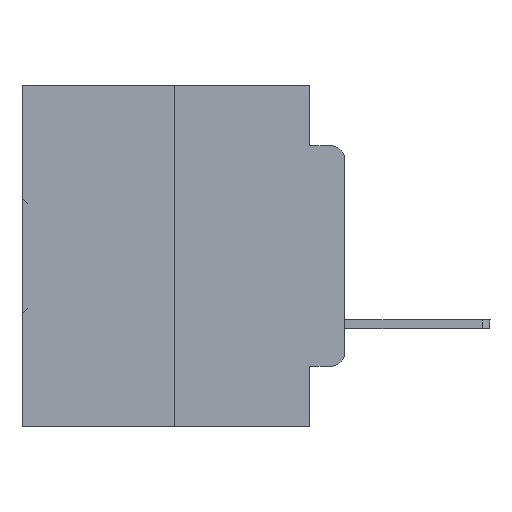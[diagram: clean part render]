
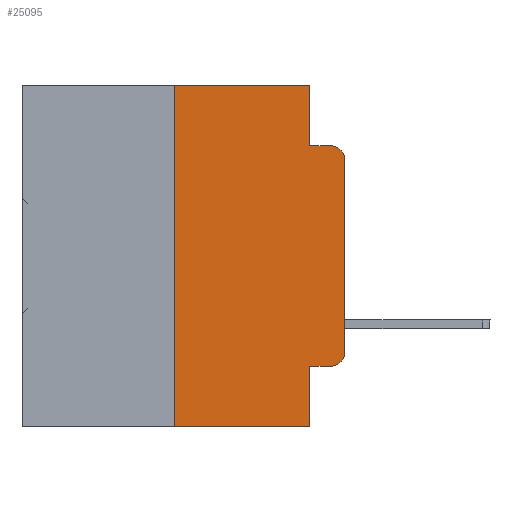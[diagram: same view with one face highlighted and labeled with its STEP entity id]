
A CAD part, left-side view. The second image highlights one B-rep face of the part: STEP entity #25095.
In plain terms, the highlighted planar face has unit normal (-1, 0, 0).
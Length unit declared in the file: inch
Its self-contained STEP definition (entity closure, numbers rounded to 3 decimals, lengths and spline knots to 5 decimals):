
#17 = VERTEX_POINT ( 'NONE', #32914 ) ;
#161 = DIRECTION ( 'NONE',  ( 0., 0., 1. ) ) ;
#197 = LINE ( 'NONE', #3133, #27004 ) ;
#233 = VERTEX_POINT ( 'NONE', #13519 ) ;
#1277 = AXIS2_PLACEMENT_3D ( 'NONE', #22930, #14975, #9777 ) ;
#1588 = CIRCLE ( 'NONE', #32548, 0.02 ) ;
#2910 = CARTESIAN_POINT ( 'NONE',  ( 0., 0.02, -0.1085 ) ) ;
#2919 = VERTEX_POINT ( 'NONE', #33240 ) ;
#2960 = CARTESIAN_POINT ( 'NONE',  ( 0., 0.25, 0. ) ) ;
#3133 = CARTESIAN_POINT ( 'NONE',  ( 0., 0., 0. ) ) ;
#3198 = VECTOR ( 'NONE', #15450, 39.37008 ) ;
#3259 = VERTEX_POINT ( 'NONE', #22315 ) ;
#3593 = EDGE_CURVE ( 'NONE', #28113, #3259, #18991, .T. ) ;
#3687 = CARTESIAN_POINT ( 'NONE',  ( 0., 0.473, 0. ) ) ;
#3763 = CARTESIAN_POINT ( 'NONE',  ( 0., 0.051, 0. ) ) ;
#4134 = CARTESIAN_POINT ( 'NONE',  ( 0., 0.051, -0.4115 ) ) ;
#4249 = AXIS2_PLACEMENT_3D ( 'NONE', #3687, #21856, #28205 ) ;
#4775 = DIRECTION ( 'NONE',  ( 0., -1., 0. ) ) ;
#5702 = CIRCLE ( 'NONE', #1277, 0.02 ) ;
#6539 = ORIENTED_EDGE ( 'NONE', *, *, #26640, .T. ) ;
#8245 = VERTEX_POINT ( 'NONE', #19595 ) ;
#8255 = EDGE_LOOP ( 'NONE', ( #6539, #17867, #20462, #9425, #28449, #27258, #11846, #21145, #8725, #27569 ) ) ;
#8432 = VERTEX_POINT ( 'NONE', #2960 ) ;
#8687 = CARTESIAN_POINT ( 'NONE',  ( 0., 0.02, -0.4115 ) ) ;
#8717 = FACE_OUTER_BOUND ( 'NONE', #8255, .T. ) ;
#8725 = ORIENTED_EDGE ( 'NONE', *, *, #16776, .T. ) ;
#9425 = ORIENTED_EDGE ( 'NONE', *, *, #13124, .F. ) ;
#9511 = EDGE_CURVE ( 'NONE', #33677, #17, #5702, .T. ) ;
#9608 = LINE ( 'NONE', #30897, #21952 ) ;
#9777 = DIRECTION ( 'NONE',  ( 0., 0., -1. ) ) ;
#9856 = LINE ( 'NONE', #20417, #18588 ) ;
#10170 = EDGE_CURVE ( 'NONE', #8245, #8432, #16103, .T. ) ;
#10611 = DIRECTION ( 'NONE',  ( 0., 0., -1. ) ) ;
#10688 = DIRECTION ( 'NONE',  ( 0., 0., -1. ) ) ;
#10712 = DIRECTION ( 'NONE',  ( 0., -1., 0. ) ) ;
#10887 = CARTESIAN_POINT ( 'NONE',  ( 0., 0.25, 0. ) ) ;
#11199 = DIRECTION ( 'NONE',  ( 0., 0., -1. ) ) ;
#11297 = PLANE ( 'NONE',  #4249 ) ;
#11846 = ORIENTED_EDGE ( 'NONE', *, *, #22435, .T. ) ;
#12479 = LINE ( 'NONE', #22522, #3198 ) ;
#13124 = EDGE_CURVE ( 'NONE', #233, #30140, #33976, .T. ) ;
#13519 = CARTESIAN_POINT ( 'NONE',  ( 0., 0.051, 0. ) ) ;
#13526 = DIRECTION ( 'NONE',  ( 0., 0., 1. ) ) ;
#13915 = CARTESIAN_POINT ( 'NONE',  ( 0., 0.02, -0.0885 ) ) ;
#14975 = DIRECTION ( 'NONE',  ( -1., 0., 0. ) ) ;
#15450 = DIRECTION ( 'NONE',  ( 0., -1., 0. ) ) ;
#16103 = LINE ( 'NONE', #10887, #29464 ) ;
#16383 = CARTESIAN_POINT ( 'NONE',  ( 0., 0.051, -0.0885 ) ) ;
#16776 = EDGE_CURVE ( 'NONE', #28113, #33677, #26479, .T. ) ;
#17619 = VECTOR ( 'NONE', #10611, 39.37008 ) ;
#17867 = ORIENTED_EDGE ( 'NONE', *, *, #28480, .T. ) ;
#18588 = VECTOR ( 'NONE', #21090, 39.37008 ) ;
#18991 = LINE ( 'NONE', #3763, #27392 ) ;
#19595 = CARTESIAN_POINT ( 'NONE',  ( 0., 0.25, -0.5 ) ) ;
#20417 = CARTESIAN_POINT ( 'NONE',  ( 0., 0.473, 0. ) ) ;
#20462 = ORIENTED_EDGE ( 'NONE', *, *, #21558, .F. ) ;
#21090 = DIRECTION ( 'NONE',  ( 0., -1., 0. ) ) ;
#21145 = ORIENTED_EDGE ( 'NONE', *, *, #3593, .F. ) ;
#21558 = EDGE_CURVE ( 'NONE', #30140, #30514, #9608, .T. ) ;
#21856 = DIRECTION ( 'NONE',  ( 1., 0., 0. ) ) ;
#21952 = VECTOR ( 'NONE', #4775, 39.37008 ) ;
#22315 = CARTESIAN_POINT ( 'NONE',  ( 0., 0.051, -0.5 ) ) ;
#22435 = EDGE_CURVE ( 'NONE', #8245, #3259, #12479, .T. ) ;
#22522 = CARTESIAN_POINT ( 'NONE',  ( 0., 0.473, -0.5 ) ) ;
#22930 = CARTESIAN_POINT ( 'NONE',  ( 0., 0.02, -0.3915 ) ) ;
#23956 = EDGE_CURVE ( 'NONE', #8432, #233, #9856, .T. ) ;
#25095 = ADVANCED_FACE ( 'NONE', ( #8717 ), #11297, .F. ) ;
#26189 = CARTESIAN_POINT ( 'NONE',  ( 0., 0.051, 0. ) ) ;
#26479 = LINE ( 'NONE', #31143, #32171 ) ;
#26640 = EDGE_CURVE ( 'NONE', #17, #2919, #197, .T. ) ;
#27004 = VECTOR ( 'NONE', #13526, 39.37008 ) ;
#27258 = ORIENTED_EDGE ( 'NONE', *, *, #10170, .F. ) ;
#27392 = VECTOR ( 'NONE', #11199, 39.37008 ) ;
#27569 = ORIENTED_EDGE ( 'NONE', *, *, #9511, .T. ) ;
#28113 = VERTEX_POINT ( 'NONE', #4134 ) ;
#28205 = DIRECTION ( 'NONE',  ( 0., 0., -1. ) ) ;
#28449 = ORIENTED_EDGE ( 'NONE', *, *, #23956, .F. ) ;
#28480 = EDGE_CURVE ( 'NONE', #2919, #30514, #1588, .T. ) ;
#29464 = VECTOR ( 'NONE', #161, 39.37008 ) ;
#30140 = VERTEX_POINT ( 'NONE', #16383 ) ;
#30514 = VERTEX_POINT ( 'NONE', #13915 ) ;
#30897 = CARTESIAN_POINT ( 'NONE',  ( 0., 0.051, -0.0885 ) ) ;
#31143 = CARTESIAN_POINT ( 'NONE',  ( 0., 0.051, -0.4115 ) ) ;
#32171 = VECTOR ( 'NONE', #10712, 39.37008 ) ;
#32509 = DIRECTION ( 'NONE',  ( -1., 0., 0. ) ) ;
#32548 = AXIS2_PLACEMENT_3D ( 'NONE', #2910, #32509, #10688 ) ;
#32914 = CARTESIAN_POINT ( 'NONE',  ( 0., 0., -0.3915 ) ) ;
#33240 = CARTESIAN_POINT ( 'NONE',  ( 0., 0., -0.1085 ) ) ;
#33677 = VERTEX_POINT ( 'NONE', #8687 ) ;
#33976 = LINE ( 'NONE', #26189, #17619 ) ;
